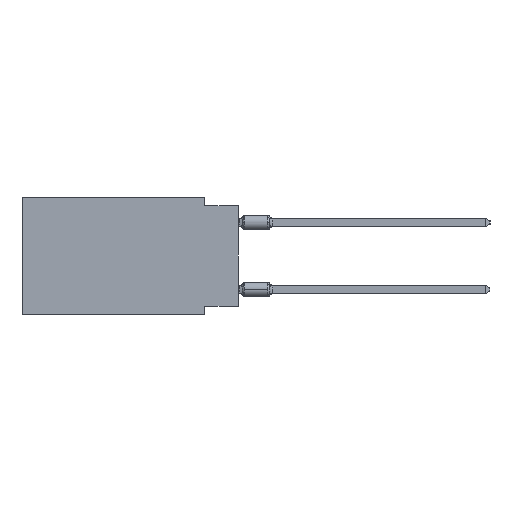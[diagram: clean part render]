
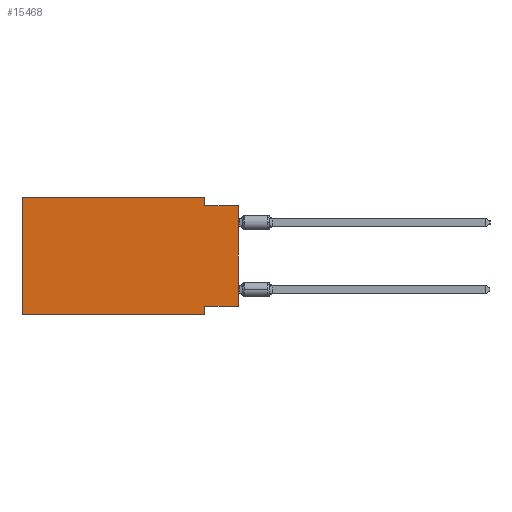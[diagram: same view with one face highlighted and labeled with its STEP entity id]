
A CAD part, left-side view. The second image highlights one B-rep face of the part: STEP entity #15468.
In plain terms, the highlighted planar face has unit normal (-1, 0, 0).
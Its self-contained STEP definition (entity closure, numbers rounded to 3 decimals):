
#435 = LINE ( 'NONE', #19885, #23921 ) ;
#1442 = DIRECTION ( 'NONE',  ( 0., 0., -1. ) ) ;
#2084 = CARTESIAN_POINT ( 'NONE',  ( 0., 16.383, -8.89 ) ) ;
#2268 = EDGE_CURVE ( 'NONE', #29833, #7361, #37085, .T. ) ;
#2578 = EDGE_CURVE ( 'NONE', #35825, #29833, #24141, .T. ) ;
#2727 = ORIENTED_EDGE ( 'NONE', *, *, #35807, .F. ) ;
#3215 = ORIENTED_EDGE ( 'NONE', *, *, #21114, .T. ) ;
#4632 = EDGE_CURVE ( 'NONE', #39290, #7361, #36388, .T. ) ;
#5031 = VECTOR ( 'NONE', #33542, 1000. ) ;
#5765 = LINE ( 'NONE', #2084, #31600 ) ;
#5771 = CARTESIAN_POINT ( 'NONE',  ( 0., 0., -0.635 ) ) ;
#7361 = VERTEX_POINT ( 'NONE', #28182 ) ;
#7836 = DIRECTION ( 'NONE',  ( 0., 0., 1. ) ) ;
#7978 = VERTEX_POINT ( 'NONE', #37183 ) ;
#8573 = CARTESIAN_POINT ( 'NONE',  ( 0., 0., -8.255 ) ) ;
#10149 = CARTESIAN_POINT ( 'NONE',  ( 0., 2.54, -8.89 ) ) ;
#10331 = LINE ( 'NONE', #34905, #24974 ) ;
#10733 = EDGE_CURVE ( 'NONE', #7978, #28979, #10331, .T. ) ;
#11621 = LINE ( 'NONE', #8573, #5031 ) ;
#11931 = VERTEX_POINT ( 'NONE', #39795 ) ;
#14337 = DIRECTION ( 'NONE',  ( 0., 0., -1. ) ) ;
#14841 = VECTOR ( 'NONE', #32937, 1000. ) ;
#14997 = AXIS2_PLACEMENT_3D ( 'NONE', #29911, #38718, #14337 ) ;
#15468 = ADVANCED_FACE ( 'NONE', ( #39114 ), #26837, .F. ) ;
#17966 = CARTESIAN_POINT ( 'NONE',  ( 0., 0., 0. ) ) ;
#18435 = EDGE_CURVE ( 'NONE', #11931, #33993, #22971, .T. ) ;
#19885 = CARTESIAN_POINT ( 'NONE',  ( 0., 16.383, 0. ) ) ;
#20854 = VECTOR ( 'NONE', #34020, 1000. ) ;
#21114 = EDGE_CURVE ( 'NONE', #11931, #28979, #5765, .T. ) ;
#21931 = ORIENTED_EDGE ( 'NONE', *, *, #2578, .F. ) ;
#22971 = LINE ( 'NONE', #23171, #38137 ) ;
#23171 = CARTESIAN_POINT ( 'NONE',  ( 0., 16.383, 0. ) ) ;
#23214 = CARTESIAN_POINT ( 'NONE',  ( 0., 16.383, 0. ) ) ;
#23325 = ORIENTED_EDGE ( 'NONE', *, *, #4632, .T. ) ;
#23921 = VECTOR ( 'NONE', #37899, 1000. ) ;
#24141 = LINE ( 'NONE', #39515, #34328 ) ;
#24349 = CARTESIAN_POINT ( 'NONE',  ( 0., 2.54, -0.635 ) ) ;
#24974 = VECTOR ( 'NONE', #31845, 1000. ) ;
#25496 = CARTESIAN_POINT ( 'NONE',  ( 0., 0., -8.255 ) ) ;
#26837 = PLANE ( 'NONE',  #14997 ) ;
#28036 = ORIENTED_EDGE ( 'NONE', *, *, #34397, .F. ) ;
#28182 = CARTESIAN_POINT ( 'NONE',  ( 0., 0., -0.635 ) ) ;
#28643 = EDGE_LOOP ( 'NONE', ( #23325, #40098, #21931, #28036, #32718, #3215, #35312, #2727 ) ) ;
#28979 = VERTEX_POINT ( 'NONE', #10149 ) ;
#29833 = VERTEX_POINT ( 'NONE', #24349 ) ;
#29911 = CARTESIAN_POINT ( 'NONE',  ( 0., 16.383, 0. ) ) ;
#30680 = CARTESIAN_POINT ( 'NONE',  ( 0., 2.54, 0. ) ) ;
#31600 = VECTOR ( 'NONE', #39956, 1000. ) ;
#31845 = DIRECTION ( 'NONE',  ( 0., 0., -1. ) ) ;
#32718 = ORIENTED_EDGE ( 'NONE', *, *, #18435, .F. ) ;
#32937 = DIRECTION ( 'NONE',  ( 0., 0., 1. ) ) ;
#33542 = DIRECTION ( 'NONE',  ( 0., 1., 0. ) ) ;
#33993 = VERTEX_POINT ( 'NONE', #23214 ) ;
#34020 = DIRECTION ( 'NONE',  ( 0., -1., 0. ) ) ;
#34328 = VECTOR ( 'NONE', #1442, 1000. ) ;
#34397 = EDGE_CURVE ( 'NONE', #33993, #35825, #435, .T. ) ;
#34905 = CARTESIAN_POINT ( 'NONE',  ( 0., 2.54, -8.89 ) ) ;
#35312 = ORIENTED_EDGE ( 'NONE', *, *, #10733, .F. ) ;
#35807 = EDGE_CURVE ( 'NONE', #39290, #7978, #11621, .T. ) ;
#35825 = VERTEX_POINT ( 'NONE', #30680 ) ;
#36388 = LINE ( 'NONE', #17966, #14841 ) ;
#37085 = LINE ( 'NONE', #5771, #20854 ) ;
#37183 = CARTESIAN_POINT ( 'NONE',  ( 0., 2.54, -8.255 ) ) ;
#37899 = DIRECTION ( 'NONE',  ( 0., -1., 0. ) ) ;
#38137 = VECTOR ( 'NONE', #7836, 1000. ) ;
#38718 = DIRECTION ( 'NONE',  ( 1., 0., 0. ) ) ;
#39114 = FACE_OUTER_BOUND ( 'NONE', #28643, .T. ) ;
#39290 = VERTEX_POINT ( 'NONE', #25496 ) ;
#39515 = CARTESIAN_POINT ( 'NONE',  ( 0., 2.54, 0. ) ) ;
#39795 = CARTESIAN_POINT ( 'NONE',  ( 0., 16.383, -8.89 ) ) ;
#39956 = DIRECTION ( 'NONE',  ( 0., -1., 0. ) ) ;
#40098 = ORIENTED_EDGE ( 'NONE', *, *, #2268, .F. ) ;
